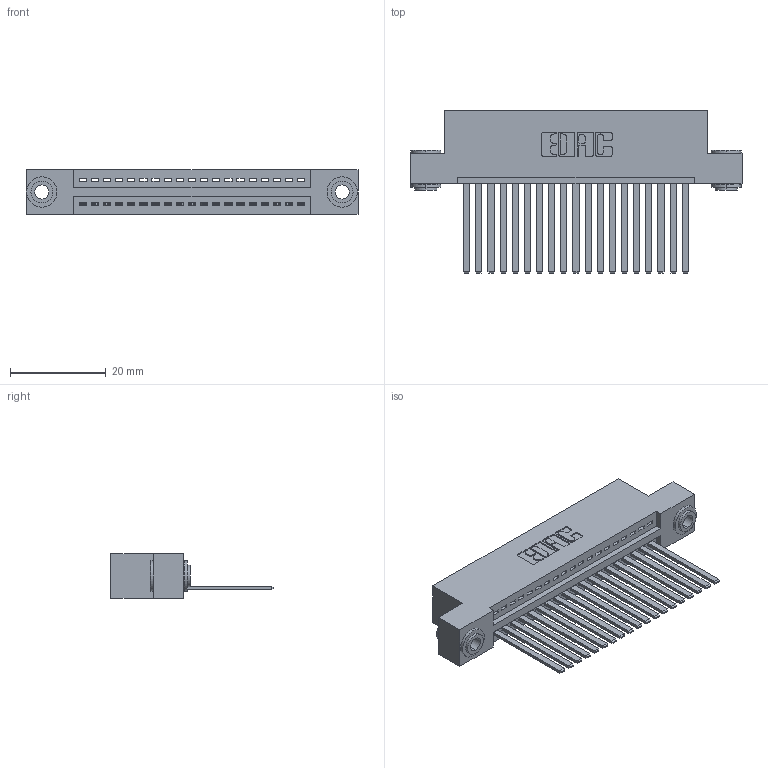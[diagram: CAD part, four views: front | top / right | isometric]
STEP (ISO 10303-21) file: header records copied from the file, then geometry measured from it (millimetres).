
FILE_DESCRIPTION (( 'STEP AP203' ), '1' );
FILE_NAME ('395-019-544-103.STEP', '2019-10-17T17:41:19', ( '' ), ( '' ), 'SwSTEP 2.0', 'SolidWorks 2016', '' );
FILE_SCHEMA (( 'CONFIG_CONTROL_DESIGN' ));
Length unit declared in the file: inch
Products named in the file (4): 395-019-544-103; 345-292-001_345-293-144; 345-250-002_345-250-002-102; 345 Part_Flush Mounting Lugs - 0.156 Dia-TH
Assembly tree (22 placements, depth 2):
  395-019-544-103
    345 Part_Flush Mounting Lugs - 0.156 Dia-TH
    345-292-001_345-293-144  x19
    345-250-002_345-250-002-102  x2
Bounding box: 69.47 x 33.96 x 9.4 mm (x, y, z)
Volume: 6649.3 mm3; surface area: 9398.8 mm2
Topology: 22 solids, 22 shells, 1152 faces, 3419 edges, 2250 vertices
Faces by surface type: plane 774, cylinder 370, cone 8
Entity records: 17862 total; most frequent: CARTESIAN_POINT 3072, ORIENTED_EDGE 3018, DIRECTION 2745, EDGE_CURVE 1509, VECTOR 1281, LINE 1281, VERTEX_POINT 1002, AXIS2_PLACEMENT_3D 732
